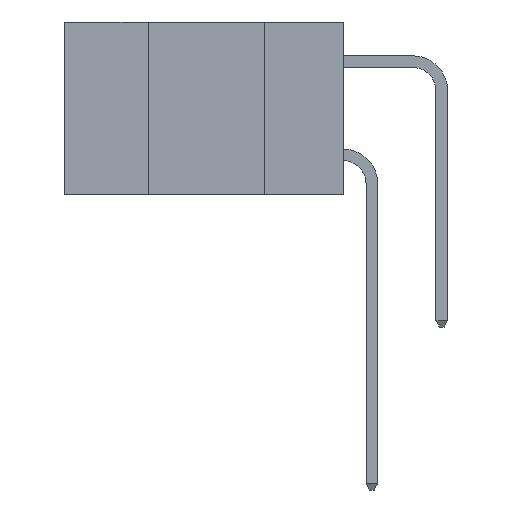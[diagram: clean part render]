
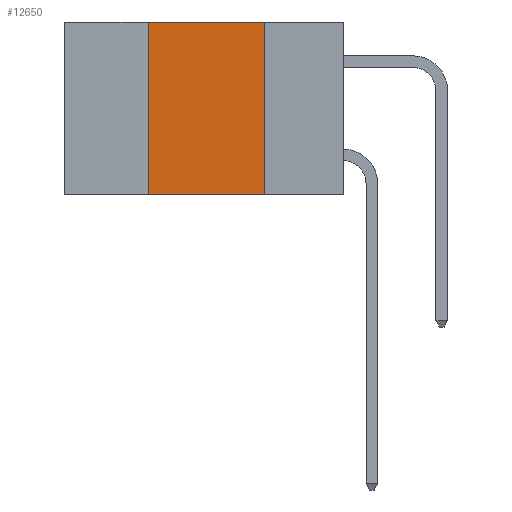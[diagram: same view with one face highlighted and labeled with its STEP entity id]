
A CAD part, left-side view. The second image highlights one B-rep face of the part: STEP entity #12650.
In plain terms, the highlighted planar face has unit normal (-1, 0, 0).
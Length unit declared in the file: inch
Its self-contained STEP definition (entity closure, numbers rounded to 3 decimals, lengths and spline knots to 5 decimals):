
#145 = EDGE_LOOP ( 'NONE', ( #15555, #7589, #2893, #5058 ) ) ;
#520 = EDGE_CURVE ( 'NONE', #8338, #12914, #3140, .T. ) ;
#637 = CARTESIAN_POINT ( 'NONE',  ( 0., 0.17, -0.37 ) ) ;
#974 = LINE ( 'NONE', #10343, #4824 ) ;
#2386 = DIRECTION ( 'NONE',  ( 0., -1., 0. ) ) ;
#2735 = EDGE_CURVE ( 'NONE', #19067, #8338, #18410, .T. ) ;
#2893 = ORIENTED_EDGE ( 'NONE', *, *, #2735, .F. ) ;
#3140 = LINE ( 'NONE', #12551, #19760 ) ;
#3885 = CARTESIAN_POINT ( 'NONE',  ( 0., 0.6, 0. ) ) ;
#4165 = DIRECTION ( 'NONE',  ( 0., 0., -1. ) ) ;
#4742 = AXIS2_PLACEMENT_3D ( 'NONE', #3885, #5505, #16734 ) ;
#4824 = VECTOR ( 'NONE', #2386, 39.37008 ) ;
#5058 = ORIENTED_EDGE ( 'NONE', *, *, #18236, .T. ) ;
#5197 = EDGE_CURVE ( 'NONE', #12914, #10655, #19045, .T. ) ;
#5505 = DIRECTION ( 'NONE',  ( 1., 0., 0. ) ) ;
#7589 = ORIENTED_EDGE ( 'NONE', *, *, #520, .F. ) ;
#7639 = CARTESIAN_POINT ( 'NONE',  ( 0., 0.17, 0. ) ) ;
#8338 = VERTEX_POINT ( 'NONE', #14880 ) ;
#10314 = CARTESIAN_POINT ( 'NONE',  ( 0., 0.42, -0.37 ) ) ;
#10343 = CARTESIAN_POINT ( 'NONE',  ( 0., 0.6, -0.37 ) ) ;
#10655 = VERTEX_POINT ( 'NONE', #637 ) ;
#11284 = DIRECTION ( 'NONE',  ( 0., -1., 0. ) ) ;
#12551 = CARTESIAN_POINT ( 'NONE',  ( 0., 0.6, 0. ) ) ;
#12650 = ADVANCED_FACE ( 'NONE', ( #14244 ), #13470, .F. ) ;
#12914 = VERTEX_POINT ( 'NONE', #7639 ) ;
#13384 = DIRECTION ( 'NONE',  ( 0., 0., 1. ) ) ;
#13460 = CARTESIAN_POINT ( 'NONE',  ( 0., 0.42, -0.37 ) ) ;
#13470 = PLANE ( 'NONE',  #4742 ) ;
#14244 = FACE_OUTER_BOUND ( 'NONE', #145, .T. ) ;
#14880 = CARTESIAN_POINT ( 'NONE',  ( 0., 0.42, 0. ) ) ;
#15555 = ORIENTED_EDGE ( 'NONE', *, *, #5197, .F. ) ;
#16734 = DIRECTION ( 'NONE',  ( 0., 0., -1. ) ) ;
#17905 = VECTOR ( 'NONE', #13384, 39.37008 ) ;
#18236 = EDGE_CURVE ( 'NONE', #19067, #10655, #974, .T. ) ;
#18410 = LINE ( 'NONE', #13460, #17905 ) ;
#18552 = VECTOR ( 'NONE', #4165, 39.37008 ) ;
#19045 = LINE ( 'NONE', #20188, #18552 ) ;
#19067 = VERTEX_POINT ( 'NONE', #10314 ) ;
#19760 = VECTOR ( 'NONE', #11284, 39.37008 ) ;
#20188 = CARTESIAN_POINT ( 'NONE',  ( 0., 0.17, -0.37 ) ) ;
